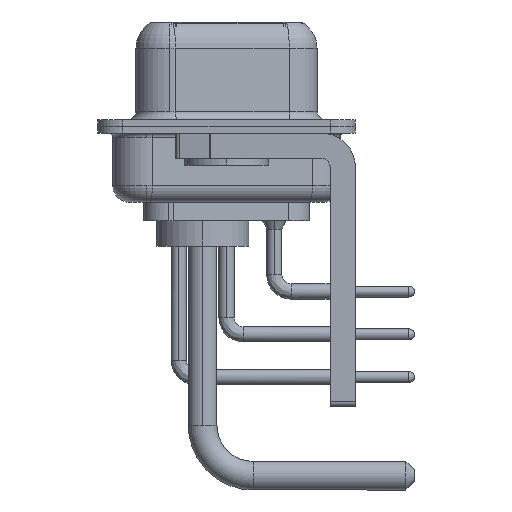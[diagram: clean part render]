
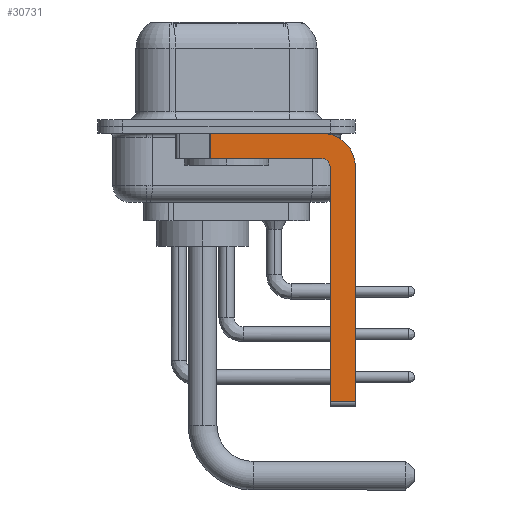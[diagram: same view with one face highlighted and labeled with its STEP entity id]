
A CAD part, left-side view. The second image highlights one B-rep face of the part: STEP entity #30731.
In plain terms, the highlighted planar face has unit normal (-1, 0, 0).
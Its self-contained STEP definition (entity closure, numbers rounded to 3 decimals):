
#1273 = CARTESIAN_POINT ( 'NONE',  ( -2.9, 3., -0.4 ) ) ;
#2038 = DIRECTION ( 'NONE',  ( 1., 0., 0. ) ) ;
#2170 = ORIENTED_EDGE ( 'NONE', *, *, #32805, .F. ) ;
#2242 = EDGE_LOOP ( 'NONE', ( #2902, #3352, #2170, #14971, #26098, #28945, #15804, #11050 ) ) ;
#2902 = ORIENTED_EDGE ( 'NONE', *, *, #21914, .F. ) ;
#3190 = EDGE_CURVE ( 'NONE', #17269, #25749, #9149, .T. ) ;
#3352 = ORIENTED_EDGE ( 'NONE', *, *, #30599, .T. ) ;
#3896 = DIRECTION ( 'NONE',  ( 0., 1., 0. ) ) ;
#3974 = DIRECTION ( 'NONE',  ( -1., 0., 0. ) ) ;
#4016 = CARTESIAN_POINT ( 'NONE',  ( -2.9, -7.65, -16.35 ) ) ;
#5149 = VECTOR ( 'NONE', #29838, 1000. ) ;
#5621 = VERTEX_POINT ( 'NONE', #17672 ) ;
#6328 = DIRECTION ( 'NONE',  ( 0., -1., 0. ) ) ;
#7136 = CARTESIAN_POINT ( 'NONE',  ( -2.9, -6.15, -2.4 ) ) ;
#7145 = VERTEX_POINT ( 'NONE', #13399 ) ;
#7409 = VERTEX_POINT ( 'NONE', #7136 ) ;
#9149 = LINE ( 'NONE', #14549, #5149 ) ;
#9990 = VECTOR ( 'NONE', #3896, 1000. ) ;
#10012 = DIRECTION ( 'NONE',  ( 0., 0., -1. ) ) ;
#10556 = CIRCLE ( 'NONE', #18631, 0.5 ) ;
#11050 = ORIENTED_EDGE ( 'NONE', *, *, #29033, .F. ) ;
#12134 = LINE ( 'NONE', #27433, #9990 ) ;
#12316 = DIRECTION ( 'NONE',  ( 0., 0., -1. ) ) ;
#13087 = EDGE_CURVE ( 'NONE', #7145, #7409, #27612, .T. ) ;
#13399 = CARTESIAN_POINT ( 'NONE',  ( -2.9, -6.15, -16.35 ) ) ;
#13635 = LINE ( 'NONE', #16340, #27385 ) ;
#13915 = DIRECTION ( 'NONE',  ( 0., 0., 1. ) ) ;
#14549 = CARTESIAN_POINT ( 'NONE',  ( -2.9, -7.65, -2.4 ) ) ;
#14853 = CARTESIAN_POINT ( 'NONE',  ( -2.9, -5.65, -2.4 ) ) ;
#14971 = ORIENTED_EDGE ( 'NONE', *, *, #21390, .F. ) ;
#15732 = DIRECTION ( 'NONE',  ( 1., 0., 0. ) ) ;
#15804 = ORIENTED_EDGE ( 'NONE', *, *, #3190, .F. ) ;
#16307 = CARTESIAN_POINT ( 'NONE',  ( -2.9, -6.15, -16.6 ) ) ;
#16340 = CARTESIAN_POINT ( 'NONE',  ( -2.9, -5.65, -16.35 ) ) ;
#16956 = LINE ( 'NONE', #1273, #27780 ) ;
#17269 = VERTEX_POINT ( 'NONE', #21778 ) ;
#17379 = AXIS2_PLACEMENT_3D ( 'NONE', #22817, #15732, #10012 ) ;
#17672 = CARTESIAN_POINT ( 'NONE',  ( -2.9, 0.978, -1.9 ) ) ;
#18104 = FACE_OUTER_BOUND ( 'NONE', #2242, .T. ) ;
#18631 = AXIS2_PLACEMENT_3D ( 'NONE', #18811, #3974, #13915 ) ;
#18811 = CARTESIAN_POINT ( 'NONE',  ( -2.9, -5.65, -2.4 ) ) ;
#18989 = VECTOR ( 'NONE', #27186, 1000. ) ;
#19993 = VERTEX_POINT ( 'NONE', #30825 ) ;
#21390 = EDGE_CURVE ( 'NONE', #7409, #19993, #10556, .T. ) ;
#21552 = DIRECTION ( 'NONE',  ( 0., -1., 0. ) ) ;
#21778 = CARTESIAN_POINT ( 'NONE',  ( -2.9, -7.65, -2.4 ) ) ;
#21914 = EDGE_CURVE ( 'NONE', #32166, #28640, #16956, .T. ) ;
#22468 = CARTESIAN_POINT ( 'NONE',  ( -2.9, -5.65, -0.4 ) ) ;
#22817 = CARTESIAN_POINT ( 'NONE',  ( -2.9, -5.65, -2.4 ) ) ;
#22977 = VECTOR ( 'NONE', #24357, 1000. ) ;
#24357 = DIRECTION ( 'NONE',  ( 0., 0., 1. ) ) ;
#24462 = CARTESIAN_POINT ( 'NONE',  ( -2.9, 0.978, -0.4 ) ) ;
#25749 = VERTEX_POINT ( 'NONE', #4016 ) ;
#25841 = CIRCLE ( 'NONE', #30130, 2. ) ;
#26098 = ORIENTED_EDGE ( 'NONE', *, *, #13087, .F. ) ;
#26131 = EDGE_CURVE ( 'NONE', #7145, #25749, #13635, .T. ) ;
#27186 = DIRECTION ( 'NONE',  ( 0., 0., -1. ) ) ;
#27385 = VECTOR ( 'NONE', #21552, 1000. ) ;
#27433 = CARTESIAN_POINT ( 'NONE',  ( -2.9, -5.65, -1.9 ) ) ;
#27612 = LINE ( 'NONE', #16307, #22977 ) ;
#27780 = VECTOR ( 'NONE', #6328, 1000. ) ;
#28340 = PLANE ( 'NONE',  #17379 ) ;
#28640 = VERTEX_POINT ( 'NONE', #22468 ) ;
#28945 = ORIENTED_EDGE ( 'NONE', *, *, #26131, .T. ) ;
#29033 = EDGE_CURVE ( 'NONE', #28640, #17269, #25841, .T. ) ;
#29838 = DIRECTION ( 'NONE',  ( 0., 0., -1. ) ) ;
#30130 = AXIS2_PLACEMENT_3D ( 'NONE', #14853, #2038, #12316 ) ;
#30359 = LINE ( 'NONE', #32259, #18989 ) ;
#30599 = EDGE_CURVE ( 'NONE', #32166, #5621, #30359, .T. ) ;
#30731 = ADVANCED_FACE ( 'NONE', ( #18104 ), #28340, .F. ) ;
#30825 = CARTESIAN_POINT ( 'NONE',  ( -2.9, -5.65, -1.9 ) ) ;
#32166 = VERTEX_POINT ( 'NONE', #24462 ) ;
#32259 = CARTESIAN_POINT ( 'NONE',  ( -2.9, 0.978, -1.9 ) ) ;
#32805 = EDGE_CURVE ( 'NONE', #19993, #5621, #12134, .T. ) ;
